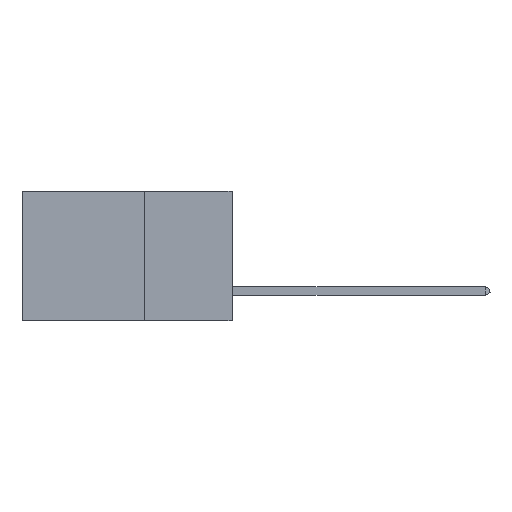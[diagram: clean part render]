
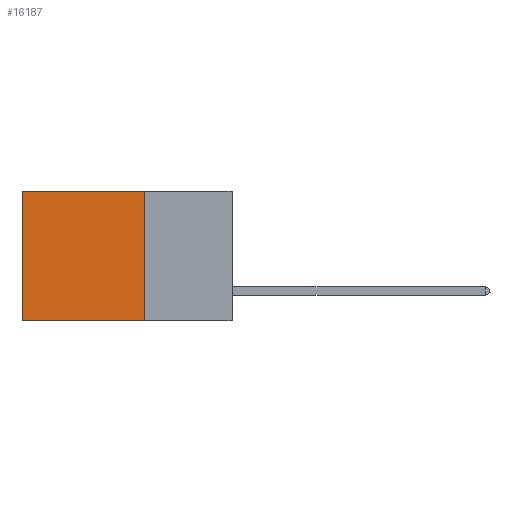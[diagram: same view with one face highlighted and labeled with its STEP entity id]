
A CAD part, left-side view. The second image highlights one B-rep face of the part: STEP entity #16187.
In plain terms, the highlighted planar face has unit normal (-1, 0, 0).
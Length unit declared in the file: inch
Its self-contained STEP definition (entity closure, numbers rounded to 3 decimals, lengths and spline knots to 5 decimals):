
#298 = CARTESIAN_POINT ( 'NONE',  ( 0.2875, 0.25, 0. ) ) ;
#2841 = CARTESIAN_POINT ( 'NONE',  ( 0.2875, 0.25, -0.37 ) ) ;
#3406 = VECTOR ( 'NONE', #6531, 39.37008 ) ;
#5076 = EDGE_LOOP ( 'NONE', ( #45241, #45307, #34796, #34931 ) ) ;
#6531 = DIRECTION ( 'NONE',  ( 0., 1., 0. ) ) ;
#6887 = LINE ( 'NONE', #38453, #49317 ) ;
#9105 = VERTEX_POINT ( 'NONE', #30126 ) ;
#10176 = LINE ( 'NONE', #298, #18667 ) ;
#14315 = CARTESIAN_POINT ( 'NONE',  ( 0.2875, 0.25, 0. ) ) ;
#16187 = ADVANCED_FACE ( 'NONE', ( #17055 ), #29788, .F. ) ;
#17055 = FACE_OUTER_BOUND ( 'NONE', #5076, .T. ) ;
#18667 = VECTOR ( 'NONE', #38753, 39.37008 ) ;
#18761 = DIRECTION ( 'NONE',  ( 0., 0., -1. ) ) ;
#19802 = EDGE_CURVE ( 'NONE', #22748, #31973, #6887, .T. ) ;
#22748 = VERTEX_POINT ( 'NONE', #27799 ) ;
#25944 = VERTEX_POINT ( 'NONE', #49075 ) ;
#26146 = EDGE_CURVE ( 'NONE', #9105, #22748, #10176, .T. ) ;
#27654 = EDGE_CURVE ( 'NONE', #9105, #25944, #42258, .T. ) ;
#27799 = CARTESIAN_POINT ( 'NONE',  ( 0.2875, 0.6, 0. ) ) ;
#28896 = CARTESIAN_POINT ( 'NONE',  ( 0.2875, 0.25, 0. ) ) ;
#28986 = VECTOR ( 'NONE', #32799, 39.37008 ) ;
#29788 = PLANE ( 'NONE',  #46238 ) ;
#30126 = CARTESIAN_POINT ( 'NONE',  ( 0.2875, 0.25, 0. ) ) ;
#30368 = CARTESIAN_POINT ( 'NONE',  ( 0.2875, 0.6, -0.37 ) ) ;
#31973 = VERTEX_POINT ( 'NONE', #30368 ) ;
#32799 = DIRECTION ( 'NONE',  ( 0., 0., -1. ) ) ;
#34796 = ORIENTED_EDGE ( 'NONE', *, *, #27654, .F. ) ;
#34931 = ORIENTED_EDGE ( 'NONE', *, *, #26146, .T. ) ;
#38453 = CARTESIAN_POINT ( 'NONE',  ( 0.2875, 0.6, 0. ) ) ;
#38753 = DIRECTION ( 'NONE',  ( 0., 1., 0. ) ) ;
#42258 = LINE ( 'NONE', #28896, #28986 ) ;
#44236 = EDGE_CURVE ( 'NONE', #25944, #31973, #50029, .T. ) ;
#44847 = DIRECTION ( 'NONE',  ( 0., 0., -1. ) ) ;
#45159 = DIRECTION ( 'NONE',  ( 1., 0., 0. ) ) ;
#45241 = ORIENTED_EDGE ( 'NONE', *, *, #19802, .T. ) ;
#45307 = ORIENTED_EDGE ( 'NONE', *, *, #44236, .F. ) ;
#46238 = AXIS2_PLACEMENT_3D ( 'NONE', #14315, #45159, #44847 ) ;
#49075 = CARTESIAN_POINT ( 'NONE',  ( 0.2875, 0.25, -0.37 ) ) ;
#49317 = VECTOR ( 'NONE', #18761, 39.37008 ) ;
#50029 = LINE ( 'NONE', #2841, #3406 ) ;
